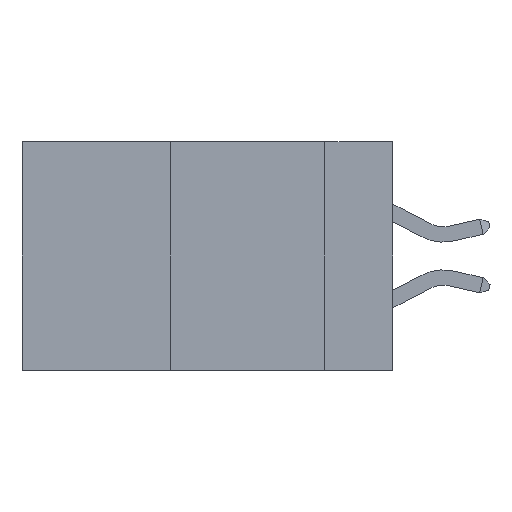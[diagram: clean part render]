
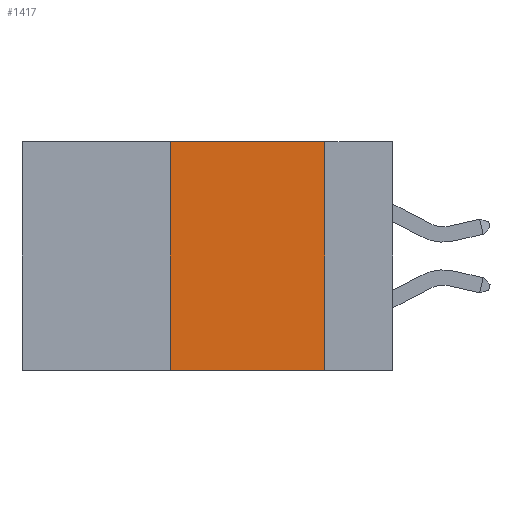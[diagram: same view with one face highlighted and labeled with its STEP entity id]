
A CAD part, left-side view. The second image highlights one B-rep face of the part: STEP entity #1417.
In plain terms, the highlighted planar face has unit normal (-1, 0, 0).
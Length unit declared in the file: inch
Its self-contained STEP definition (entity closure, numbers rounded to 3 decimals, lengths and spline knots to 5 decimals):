
#110 = VECTOR ( 'NONE', #303, 39.37008 ) ;
#303 = DIRECTION ( 'NONE',  ( 0., -1., 0. ) ) ;
#311 = VECTOR ( 'NONE', #12993, 39.37008 ) ;
#629 = LINE ( 'NONE', #8881, #15771 ) ;
#805 = ORIENTED_EDGE ( 'NONE', *, *, #10340, .F. ) ;
#876 = FACE_OUTER_BOUND ( 'NONE', #1725, .T. ) ;
#1417 = ADVANCED_FACE ( 'NONE', ( #876 ), #14498, .F. ) ;
#1725 = EDGE_LOOP ( 'NONE', ( #3171, #805, #9892, #9213 ) ) ;
#3171 = ORIENTED_EDGE ( 'NONE', *, *, #6084, .F. ) ;
#3348 = VERTEX_POINT ( 'NONE', #6691 ) ;
#4027 = LINE ( 'NONE', #5883, #110 ) ;
#4207 = CARTESIAN_POINT ( 'NONE',  ( 0., 0.6, 0. ) ) ;
#4334 = EDGE_CURVE ( 'NONE', #3348, #17005, #629, .T. ) ;
#5822 = LINE ( 'NONE', #10345, #11153 ) ;
#5883 = CARTESIAN_POINT ( 'NONE',  ( 0., 0.6, 0. ) ) ;
#6084 = EDGE_CURVE ( 'NONE', #11198, #16579, #5822, .T. ) ;
#6510 = LINE ( 'NONE', #15553, #311 ) ;
#6691 = CARTESIAN_POINT ( 'NONE',  ( 0., 0.36, -0.37 ) ) ;
#8598 = CARTESIAN_POINT ( 'NONE',  ( 0., 0.36, 0. ) ) ;
#8881 = CARTESIAN_POINT ( 'NONE',  ( 0., 0.36, 0. ) ) ;
#9213 = ORIENTED_EDGE ( 'NONE', *, *, #18984, .T. ) ;
#9892 = ORIENTED_EDGE ( 'NONE', *, *, #4334, .F. ) ;
#9975 = DIRECTION ( 'NONE',  ( 1., 0., 0. ) ) ;
#10145 = CARTESIAN_POINT ( 'NONE',  ( 0., 0.11, 0. ) ) ;
#10340 = EDGE_CURVE ( 'NONE', #17005, #11198, #4027, .T. ) ;
#10345 = CARTESIAN_POINT ( 'NONE',  ( 0., 0.11, 0. ) ) ;
#10435 = DIRECTION ( 'NONE',  ( 0., 0., 1. ) ) ;
#10949 = AXIS2_PLACEMENT_3D ( 'NONE', #4207, #9975, #15819 ) ;
#11153 = VECTOR ( 'NONE', #16939, 39.37008 ) ;
#11198 = VERTEX_POINT ( 'NONE', #10145 ) ;
#12993 = DIRECTION ( 'NONE',  ( 0., -1., 0. ) ) ;
#14498 = PLANE ( 'NONE',  #10949 ) ;
#14839 = CARTESIAN_POINT ( 'NONE',  ( 0., 0.11, -0.37 ) ) ;
#15553 = CARTESIAN_POINT ( 'NONE',  ( 0., 0.6, -0.37 ) ) ;
#15771 = VECTOR ( 'NONE', #10435, 39.37008 ) ;
#15819 = DIRECTION ( 'NONE',  ( 0., 0., -1. ) ) ;
#16579 = VERTEX_POINT ( 'NONE', #14839 ) ;
#16939 = DIRECTION ( 'NONE',  ( 0., 0., -1. ) ) ;
#17005 = VERTEX_POINT ( 'NONE', #8598 ) ;
#18984 = EDGE_CURVE ( 'NONE', #3348, #16579, #6510, .T. ) ;
